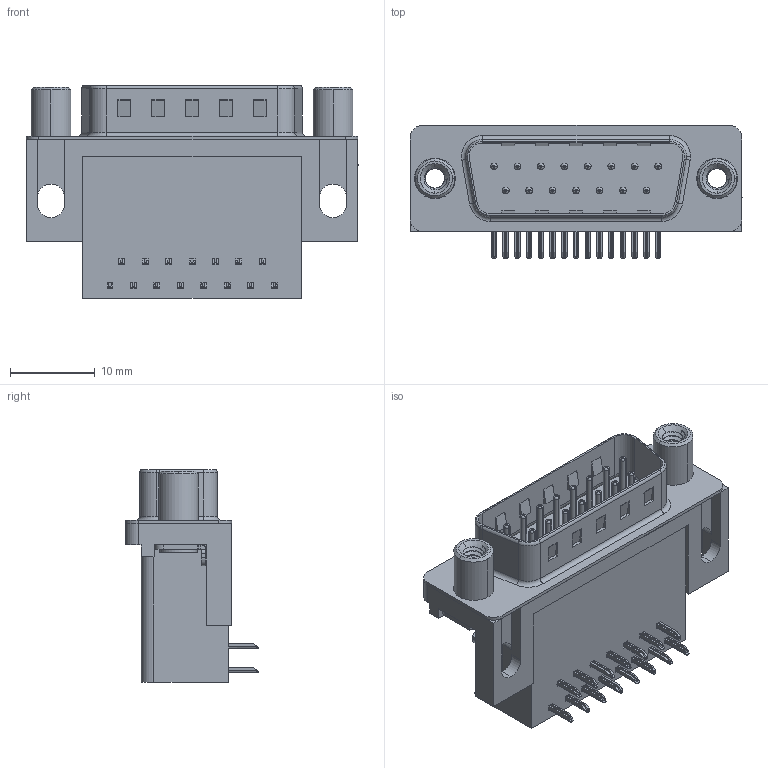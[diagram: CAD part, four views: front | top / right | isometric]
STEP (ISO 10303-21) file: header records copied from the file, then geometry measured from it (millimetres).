
FILE_DESCRIPTION (( 'STEP AP203' ), '1' );
FILE_NAME ('625-015-362-000.STEP', '2018-11-05T23:10:01', ( '' ), ( '' ), 'SwSTEP 2.0', 'SolidWorks 2016', '' );
FILE_SCHEMA (( 'CONFIG_CONTROL_DESIGN' ));
Length unit declared in the file: millimetre
Products named in the file (7): 625 Contact Top; 625-015-362-000; 625 Shell_15 Socket; 625 Non Board Mount; 625 Housing_15 Socket; 625 Round Threaded Standoff; 625 Contact Bottom
Assembly tree (21 placements, depth 2):
  625-015-362-000
    625 Housing_15 Socket
    625 Shell_15 Socket
    625 Contact Bottom  x7
    625 Contact Top  x8
    625 Non Board Mount  x2
    625 Round Threaded Standoff  x2
Bounding box: 39.22 x 15.73 x 25.16 mm (x, y, z)
Volume: 6305.6 mm3; surface area: 6489.6 mm2
Topology: 21 solids, 21 shells, 1471 faces, 3677 edges, 2283 vertices
Faces by surface type: plane 887, cylinder 451, torus 105, bspline 16, cone 12
Entity records: 19089 total; most frequent: CARTESIAN_POINT 4758, DIRECTION 2772, ORIENTED_EDGE 2710, EDGE_CURVE 1355, AXIS2_PLACEMENT_3D 929, VECTOR 914, LINE 914, VERTEX_POINT 867
